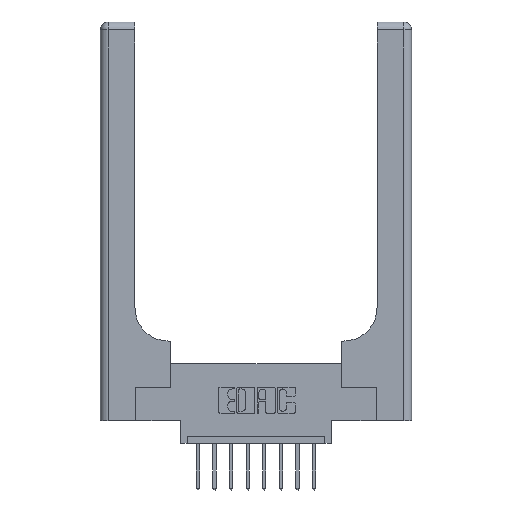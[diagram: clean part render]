
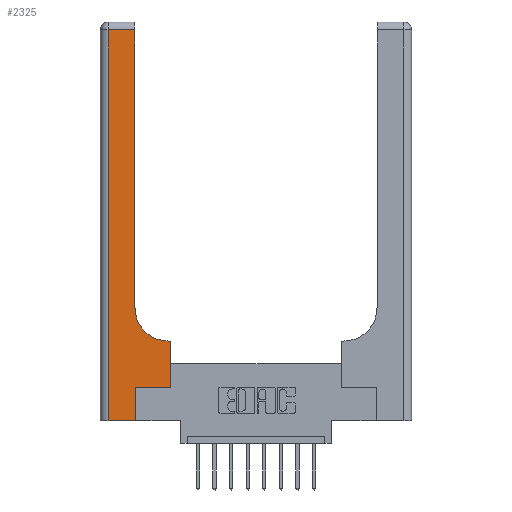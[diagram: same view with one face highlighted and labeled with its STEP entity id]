
A CAD part, top view. The second image highlights one B-rep face of the part: STEP entity #2325.
In plain terms, the highlighted planar face has unit normal (0, 0, 1).
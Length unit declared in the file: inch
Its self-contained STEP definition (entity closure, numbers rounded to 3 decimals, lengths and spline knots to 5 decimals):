
#78 = AXIS2_PLACEMENT_3D ( 'NONE', #11123, #508, #432 ) ;
#366 = VERTEX_POINT ( 'NONE', #1945 ) ;
#432 = DIRECTION ( 'NONE',  ( -1., 0., 0. ) ) ;
#508 = DIRECTION ( 'NONE',  ( 0., 0., -1. ) ) ;
#660 = CARTESIAN_POINT ( 'NONE',  ( 0.26, 2.94, 0.37 ) ) ;
#734 = CARTESIAN_POINT ( 'NONE',  ( 0., 0., 0.37 ) ) ;
#1311 = DIRECTION ( 'NONE',  ( 0., 0., -1. ) ) ;
#1514 = VERTEX_POINT ( 'NONE', #3032 ) ;
#1615 = CIRCLE ( 'NONE', #14214, 0.25 ) ;
#1945 = CARTESIAN_POINT ( 'NONE',  ( 0.528, 0.25, 0.37 ) ) ;
#2120 = EDGE_LOOP ( 'NONE', ( #5664, #8760, #12524, #11843, #5050, #14750, #6687, #11836, #7341 ) ) ;
#2325 = ADVANCED_FACE ( 'NONE', ( #13612 ), #13460, .F. ) ;
#2349 = DIRECTION ( 'NONE',  ( 0., 1., 0. ) ) ;
#2920 = VERTEX_POINT ( 'NONE', #12523 ) ;
#3032 = CARTESIAN_POINT ( 'NONE',  ( 0.528, 0.6, 0.37 ) ) ;
#3422 = VERTEX_POINT ( 'NONE', #13956 ) ;
#3595 = CARTESIAN_POINT ( 'NONE',  ( 0., 2.94, 0.37 ) ) ;
#3808 = LINE ( 'NONE', #13431, #5188 ) ;
#3850 = CARTESIAN_POINT ( 'NONE',  ( 0.26, 3., 0.37 ) ) ;
#3999 = VECTOR ( 'NONE', #14283, 39.37008 ) ;
#4221 = DIRECTION ( 'NONE',  ( 1., 0., 0. ) ) ;
#4856 = LINE ( 'NONE', #3850, #9253 ) ;
#5050 = ORIENTED_EDGE ( 'NONE', *, *, #5168, .T. ) ;
#5168 = EDGE_CURVE ( 'NONE', #2920, #10689, #13943, .T. ) ;
#5188 = VECTOR ( 'NONE', #13508, 39.37008 ) ;
#5237 = EDGE_CURVE ( 'NONE', #3422, #8821, #1615, .T. ) ;
#5250 = VERTEX_POINT ( 'NONE', #13258 ) ;
#5313 = EDGE_CURVE ( 'NONE', #8821, #12215, #4856, .T. ) ;
#5610 = LINE ( 'NONE', #10703, #11893 ) ;
#5664 = ORIENTED_EDGE ( 'NONE', *, *, #5313, .T. ) ;
#5698 = CARTESIAN_POINT ( 'NONE',  ( 0.26, 0.85, 0.37 ) ) ;
#6047 = EDGE_CURVE ( 'NONE', #10689, #366, #8136, .T. ) ;
#6185 = VECTOR ( 'NONE', #4221, 39.37008 ) ;
#6687 = ORIENTED_EDGE ( 'NONE', *, *, #13860, .T. ) ;
#7259 = CARTESIAN_POINT ( 'NONE',  ( 0.265, 0.25, 0.37 ) ) ;
#7285 = VECTOR ( 'NONE', #13025, 39.37008 ) ;
#7341 = ORIENTED_EDGE ( 'NONE', *, *, #5237, .T. ) ;
#8047 = EDGE_CURVE ( 'NONE', #1514, #3422, #5610, .T. ) ;
#8136 = LINE ( 'NONE', #11435, #14741 ) ;
#8151 = EDGE_CURVE ( 'NONE', #8237, #5250, #3808, .T. ) ;
#8237 = VERTEX_POINT ( 'NONE', #10939 ) ;
#8251 = CARTESIAN_POINT ( 'NONE',  ( 0.265, 0., 0.37 ) ) ;
#8273 = CARTESIAN_POINT ( 'NONE',  ( 0.528, 0.25, 0.37 ) ) ;
#8395 = DIRECTION ( 'NONE',  ( 1., 0., 0. ) ) ;
#8760 = ORIENTED_EDGE ( 'NONE', *, *, #15169, .T. ) ;
#8821 = VERTEX_POINT ( 'NONE', #5698 ) ;
#9253 = VECTOR ( 'NONE', #9876, 39.37008 ) ;
#9538 = LINE ( 'NONE', #3595, #3999 ) ;
#9876 = DIRECTION ( 'NONE',  ( 0., 1., 0. ) ) ;
#10154 = VECTOR ( 'NONE', #2349, 39.37008 ) ;
#10689 = VERTEX_POINT ( 'NONE', #7259 ) ;
#10703 = CARTESIAN_POINT ( 'NONE',  ( 0.26, 0.6, 0.37 ) ) ;
#10939 = CARTESIAN_POINT ( 'NONE',  ( 0.06, 2.94, 0.37 ) ) ;
#11123 = CARTESIAN_POINT ( 'NONE',  ( 0., 3., 0.37 ) ) ;
#11435 = CARTESIAN_POINT ( 'NONE',  ( 0.265, 0.25, 0.37 ) ) ;
#11836 = ORIENTED_EDGE ( 'NONE', *, *, #8047, .T. ) ;
#11843 = ORIENTED_EDGE ( 'NONE', *, *, #13328, .T. ) ;
#11893 = VECTOR ( 'NONE', #13209, 39.37008 ) ;
#12215 = VERTEX_POINT ( 'NONE', #660 ) ;
#12523 = CARTESIAN_POINT ( 'NONE',  ( 0.265, 0., 0.37 ) ) ;
#12524 = ORIENTED_EDGE ( 'NONE', *, *, #8151, .T. ) ;
#12762 = DIRECTION ( 'NONE',  ( 1., 0., 0. ) ) ;
#13025 = DIRECTION ( 'NONE',  ( 0., 1., 0. ) ) ;
#13209 = DIRECTION ( 'NONE',  ( -1., 0., 0. ) ) ;
#13258 = CARTESIAN_POINT ( 'NONE',  ( 0.06, 0., 0.37 ) ) ;
#13325 = CARTESIAN_POINT ( 'NONE',  ( 0.51, 0.85, 0.37 ) ) ;
#13328 = EDGE_CURVE ( 'NONE', #5250, #2920, #13616, .T. ) ;
#13431 = CARTESIAN_POINT ( 'NONE',  ( 0.06, 3., 0.37 ) ) ;
#13460 = PLANE ( 'NONE',  #78 ) ;
#13508 = DIRECTION ( 'NONE',  ( 0., -1., 0. ) ) ;
#13612 = FACE_OUTER_BOUND ( 'NONE', #2120, .T. ) ;
#13616 = LINE ( 'NONE', #734, #6185 ) ;
#13860 = EDGE_CURVE ( 'NONE', #366, #1514, #14190, .T. ) ;
#13943 = LINE ( 'NONE', #8251, #7285 ) ;
#13956 = CARTESIAN_POINT ( 'NONE',  ( 0.51, 0.6, 0.37 ) ) ;
#14190 = LINE ( 'NONE', #8273, #10154 ) ;
#14214 = AXIS2_PLACEMENT_3D ( 'NONE', #13325, #1311, #8395 ) ;
#14283 = DIRECTION ( 'NONE',  ( -1., 0., 0. ) ) ;
#14741 = VECTOR ( 'NONE', #12762, 39.37008 ) ;
#14750 = ORIENTED_EDGE ( 'NONE', *, *, #6047, .T. ) ;
#15169 = EDGE_CURVE ( 'NONE', #12215, #8237, #9538, .T. ) ;
